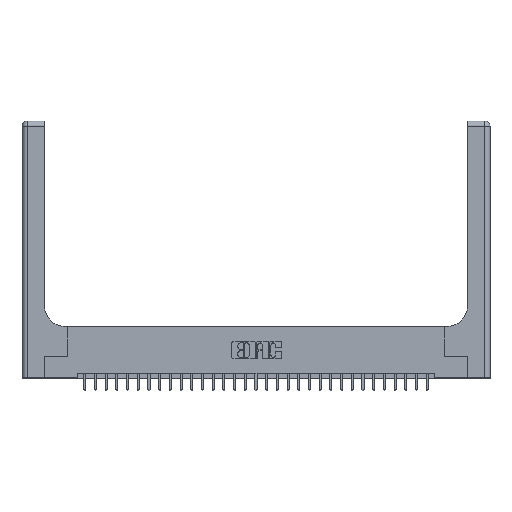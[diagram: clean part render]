
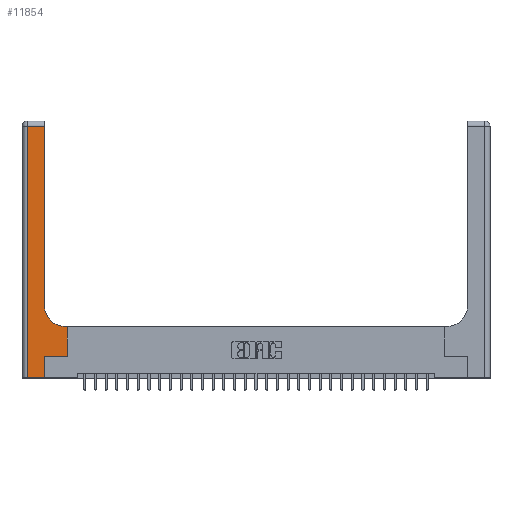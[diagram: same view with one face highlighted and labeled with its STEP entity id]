
A CAD part, top view. The second image highlights one B-rep face of the part: STEP entity #11854.
In plain terms, the highlighted planar face has unit normal (0, 0, 1).
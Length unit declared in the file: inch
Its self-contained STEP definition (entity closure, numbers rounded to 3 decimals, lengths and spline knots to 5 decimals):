
#324 = VECTOR ( 'NONE', #21799, 39.37008 ) ;
#996 = CARTESIAN_POINT ( 'NONE',  ( 0.265, 0.25, 0.37 ) ) ;
#1165 = CARTESIAN_POINT ( 'NONE',  ( 0.51, 0.6, 0.37 ) ) ;
#2008 = VERTEX_POINT ( 'NONE', #16164 ) ;
#2887 = ORIENTED_EDGE ( 'NONE', *, *, #13822, .T. ) ;
#2921 = EDGE_CURVE ( 'NONE', #6930, #8447, #22422, .T. ) ;
#3412 = EDGE_CURVE ( 'NONE', #5627, #22444, #7603, .T. ) ;
#3466 = DIRECTION ( 'NONE',  ( -1., 0., 0. ) ) ;
#3821 = EDGE_CURVE ( 'NONE', #2008, #4488, #22429, .T. ) ;
#3860 = VECTOR ( 'NONE', #20054, 39.37008 ) ;
#4276 = LINE ( 'NONE', #25673, #19128 ) ;
#4485 = VECTOR ( 'NONE', #3466, 39.37008 ) ;
#4488 = VERTEX_POINT ( 'NONE', #14461 ) ;
#4924 = AXIS2_PLACEMENT_3D ( 'NONE', #23164, #10340, #12700 ) ;
#5309 = LINE ( 'NONE', #8329, #20510 ) ;
#5403 = VERTEX_POINT ( 'NONE', #10965 ) ;
#5627 = VERTEX_POINT ( 'NONE', #27101 ) ;
#5972 = CARTESIAN_POINT ( 'NONE',  ( 0.528, 0.6, 0.37 ) ) ;
#6518 = VECTOR ( 'NONE', #9665, 39.37008 ) ;
#6930 = VERTEX_POINT ( 'NONE', #24889 ) ;
#6934 = CARTESIAN_POINT ( 'NONE',  ( 0., 0., 0.37 ) ) ;
#7364 = ORIENTED_EDGE ( 'NONE', *, *, #11010, .T. ) ;
#7603 = LINE ( 'NONE', #13164, #27805 ) ;
#8329 = CARTESIAN_POINT ( 'NONE',  ( 0.06, 3., 0.37 ) ) ;
#8447 = VERTEX_POINT ( 'NONE', #11634 ) ;
#8692 = EDGE_CURVE ( 'NONE', #22444, #5403, #4276, .T. ) ;
#8876 = DIRECTION ( 'NONE',  ( 0., 1., 0. ) ) ;
#9173 = DIRECTION ( 'NONE',  ( 1., 0., 0. ) ) ;
#9184 = ORIENTED_EDGE ( 'NONE', *, *, #3412, .T. ) ;
#9369 = ORIENTED_EDGE ( 'NONE', *, *, #2921, .T. ) ;
#9665 = DIRECTION ( 'NONE',  ( 0., 1., 0. ) ) ;
#10340 = DIRECTION ( 'NONE',  ( 0., 0., -1. ) ) ;
#10698 = CARTESIAN_POINT ( 'NONE',  ( 0.26, 2.94, 0.37 ) ) ;
#10809 = VERTEX_POINT ( 'NONE', #5972 ) ;
#10965 = CARTESIAN_POINT ( 'NONE',  ( 0.06, 2.94, 0.37 ) ) ;
#11010 = EDGE_CURVE ( 'NONE', #10809, #25558, #16650, .T. ) ;
#11634 = CARTESIAN_POINT ( 'NONE',  ( 0.265, 0., 0.37 ) ) ;
#11854 = ADVANCED_FACE ( 'NONE', ( #14888 ), #21209, .F. ) ;
#12014 = EDGE_CURVE ( 'NONE', #8447, #2008, #27030, .T. ) ;
#12281 = LINE ( 'NONE', #22592, #6518 ) ;
#12700 = DIRECTION ( 'NONE',  ( 1., 0., 0. ) ) ;
#13021 = CARTESIAN_POINT ( 'NONE',  ( 0.26, 0.6, 0.37 ) ) ;
#13164 = CARTESIAN_POINT ( 'NONE',  ( 0.26, 3., 0.37 ) ) ;
#13272 = DIRECTION ( 'NONE',  ( 0., 0., -1. ) ) ;
#13822 = EDGE_CURVE ( 'NONE', #25558, #5627, #26589, .T. ) ;
#14461 = CARTESIAN_POINT ( 'NONE',  ( 0.528, 0.25, 0.37 ) ) ;
#14477 = ORIENTED_EDGE ( 'NONE', *, *, #17807, .T. ) ;
#14642 = ORIENTED_EDGE ( 'NONE', *, *, #12014, .T. ) ;
#14888 = FACE_OUTER_BOUND ( 'NONE', #24656, .T. ) ;
#15026 = VECTOR ( 'NONE', #9173, 39.37008 ) ;
#15307 = ORIENTED_EDGE ( 'NONE', *, *, #8692, .T. ) ;
#16164 = CARTESIAN_POINT ( 'NONE',  ( 0.265, 0.25, 0.37 ) ) ;
#16650 = LINE ( 'NONE', #13021, #4485 ) ;
#17788 = CARTESIAN_POINT ( 'NONE',  ( 0., 3., 0.37 ) ) ;
#17807 = EDGE_CURVE ( 'NONE', #5403, #6930, #5309, .T. ) ;
#19097 = CARTESIAN_POINT ( 'NONE',  ( 0.265, 0., 0.37 ) ) ;
#19128 = VECTOR ( 'NONE', #27928, 39.37008 ) ;
#20054 = DIRECTION ( 'NONE',  ( 1., 0., 0. ) ) ;
#20510 = VECTOR ( 'NONE', #21378, 39.37008 ) ;
#21209 = PLANE ( 'NONE',  #23510 ) ;
#21378 = DIRECTION ( 'NONE',  ( 0., -1., 0. ) ) ;
#21799 = DIRECTION ( 'NONE',  ( 0., 1., 0. ) ) ;
#22422 = LINE ( 'NONE', #6934, #3860 ) ;
#22429 = LINE ( 'NONE', #996, #15026 ) ;
#22444 = VERTEX_POINT ( 'NONE', #10698 ) ;
#22592 = CARTESIAN_POINT ( 'NONE',  ( 0.528, 0.25, 0.37 ) ) ;
#23164 = CARTESIAN_POINT ( 'NONE',  ( 0.51, 0.85, 0.37 ) ) ;
#23510 = AXIS2_PLACEMENT_3D ( 'NONE', #17788, #13272, #23927 ) ;
#23682 = EDGE_CURVE ( 'NONE', #4488, #10809, #12281, .T. ) ;
#23927 = DIRECTION ( 'NONE',  ( -1., 0., 0. ) ) ;
#24656 = EDGE_LOOP ( 'NONE', ( #9184, #15307, #14477, #9369, #14642, #25755, #26092, #7364, #2887 ) ) ;
#24889 = CARTESIAN_POINT ( 'NONE',  ( 0.06, 0., 0.37 ) ) ;
#25558 = VERTEX_POINT ( 'NONE', #1165 ) ;
#25673 = CARTESIAN_POINT ( 'NONE',  ( 0., 2.94, 0.37 ) ) ;
#25755 = ORIENTED_EDGE ( 'NONE', *, *, #3821, .T. ) ;
#26092 = ORIENTED_EDGE ( 'NONE', *, *, #23682, .T. ) ;
#26589 = CIRCLE ( 'NONE', #4924, 0.25 ) ;
#27030 = LINE ( 'NONE', #19097, #324 ) ;
#27101 = CARTESIAN_POINT ( 'NONE',  ( 0.26, 0.85, 0.37 ) ) ;
#27805 = VECTOR ( 'NONE', #8876, 39.37008 ) ;
#27928 = DIRECTION ( 'NONE',  ( -1., 0., 0. ) ) ;
